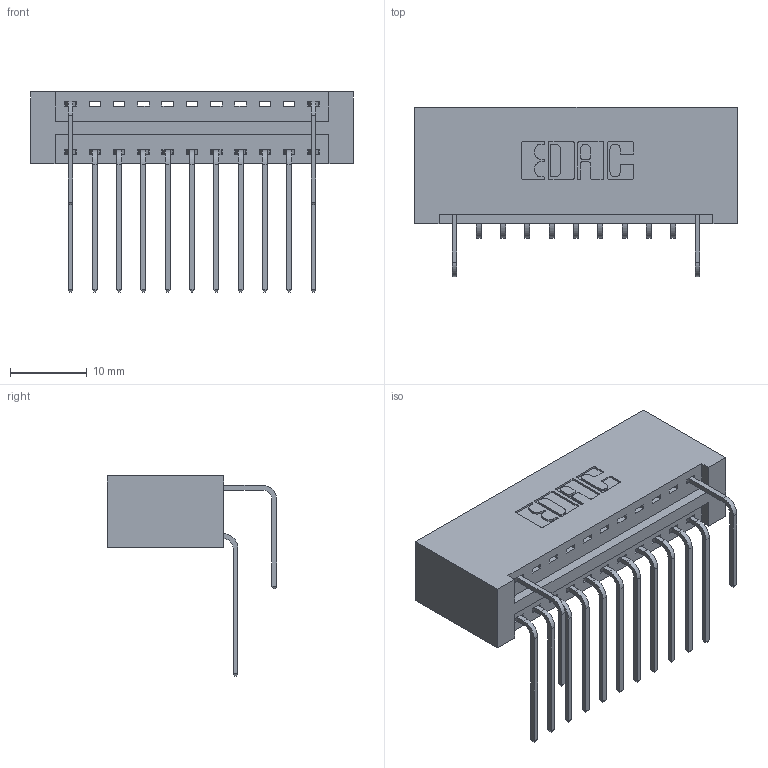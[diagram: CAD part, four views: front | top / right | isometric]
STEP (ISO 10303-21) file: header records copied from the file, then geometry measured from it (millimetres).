
FILE_DESCRIPTION (( 'STEP AP203' ), '1' );
FILE_NAME ('346-022-558-201.STEP', '2018-08-21T01:02:17', ( '' ), ( '' ), 'SwSTEP 2.0', 'SolidWorks 2016', '' );
FILE_SCHEMA (( 'CONFIG_CONTROL_DESIGN' ));
Length unit declared in the file: inch
Products named in the file (4): 345-292-001_558 559 Tail - 1; 345-292-001_558 Tail - 2; 346-022-558-201; 346 Part_No Mounting Lugs
Assembly tree (14 placements, depth 2):
  346-022-558-201
    346 Part_No Mounting Lugs
    345-292-001_558 559 Tail - 1  x11
    345-292-001_558 Tail - 2  x2
Bounding box: 42.16 x 22.16 x 26.16 mm (x, y, z)
Volume: 4438 mm3; surface area: 5669 mm2
Topology: 14 solids, 14 shells, 870 faces, 2587 edges, 1706 vertices
Faces by surface type: plane 598, cylinder 272
Entity records: 12571 total; most frequent: CARTESIAN_POINT 2202, ORIENTED_EDGE 2094, DIRECTION 1949, EDGE_CURVE 1047, LINE 839, VECTOR 839, VERTEX_POINT 694, AXIS2_PLACEMENT_3D 555
